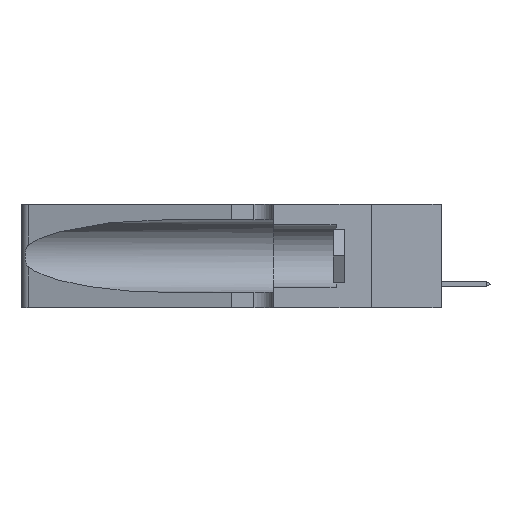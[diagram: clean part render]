
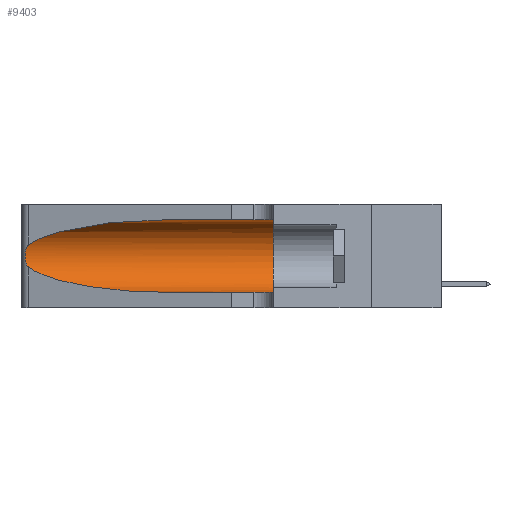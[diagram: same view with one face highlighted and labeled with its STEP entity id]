
A CAD part, left-side view. The second image highlights one B-rep face of the part: STEP entity #9403.
In plain terms, the highlighted cylindrical face has radius 3.308 mm (diameter 6.617 mm), a partial arc.
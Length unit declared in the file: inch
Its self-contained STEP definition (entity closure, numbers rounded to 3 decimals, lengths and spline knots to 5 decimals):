
#260 = DIRECTION ( 'NONE',  ( 0., 0., -1. ) ) ;
#383 = CARTESIAN_POINT ( 'NONE',  ( 0.1305, 0.35, 0.05475 ) ) ;
#609 = LINE ( 'NONE', #6390, #15550 ) ;
#777 = CARTESIAN_POINT ( 'NONE',  ( 0.2373, 1.15595, 0.28018 ) ) ;
#823 = EDGE_LOOP ( 'NONE', ( #16507, #5935, #15226, #9526, #3010, #2680 ) ) ;
#886 = EDGE_CURVE ( 'NONE', #3134, #11566, #5844, .T. ) ;
#1057 = AXIS2_PLACEMENT_3D ( 'NONE', #7533, #6177, #260 ) ;
#1418 = EDGE_CURVE ( 'NONE', #15803, #8553, #6634, .T. ) ;
#2193 = CARTESIAN_POINT ( 'NONE',  ( 0.25639, 1.23186, 0.15144 ) ) ;
#2226 = DIRECTION ( 'NONE',  ( 0., -1., 0. ) ) ;
#2521 = CYLINDRICAL_SURFACE ( 'NONE', #1057, 0.13025 ) ;
#2680 = ORIENTED_EDGE ( 'NONE', *, *, #7318, .F. ) ;
#3010 = ORIENTED_EDGE ( 'NONE', *, *, #6747, .F. ) ;
#3134 = VERTEX_POINT ( 'NONE', #3547 ) ;
#3521 = CARTESIAN_POINT ( 'NONE',  ( 0.25487, 1.22718, 0.22369 ) ) ;
#3547 = CARTESIAN_POINT ( 'NONE',  ( 0.25487, 1.22718, 0.14631 ) ) ;
#3558 = B_SPLINE_CURVE_WITH_KNOTS ( 'NONE', 3,
 ( #6538, #3743, #10888, #3803, #13723, #5171, #15155, #5228, #7777, #6603, #16568, #2193, #14972, #12322 ),
 .UNSPECIFIED., .F., .F.,
 ( 4, 2, 2, 2, 2, 2, 4 ),
 ( 0., 0.00027, 0.00053, 0.00107, 0.0016, 0.00187, 0.00214 ),
 .UNSPECIFIED. ) ;
#3738 = CARTESIAN_POINT ( 'NONE',  ( 0.1305, 0.72297, 0.05475 ) ) ;
#3743 = CARTESIAN_POINT ( 'NONE',  ( 0.25555, 1.22994, 0.2215 ) ) ;
#3803 = CARTESIAN_POINT ( 'NONE',  ( 0.25787, 1.23484, 0.2124 ) ) ;
#5097 = DIRECTION ( 'NONE',  ( 0., 0., 1. ) ) ;
#5171 = CARTESIAN_POINT ( 'NONE',  ( 0.26018, 1.23835, 0.19895 ) ) ;
#5228 = CARTESIAN_POINT ( 'NONE',  ( 0.26075, 1.23896, 0.178 ) ) ;
#5332 = CARTESIAN_POINT ( 'NONE',  ( 0.25487, 1.22718, 0.14631 ) ) ;
#5844 =( BOUNDED_CURVE ( )  B_SPLINE_CURVE ( 3, ( #5332, #10871, #15373, #6585 ),
 .UNSPECIFIED., .F., .F. ) 
 B_SPLINE_CURVE_WITH_KNOTS ( ( 4, 4 ),
 ( 3.44316, 4.71239 ),
 .UNSPECIFIED. ) 
 CURVE ( )  GEOMETRIC_REPRESENTATION_ITEM ( )  RATIONAL_B_SPLINE_CURVE ( ( 1., 0.87, 0.87, 1. ) ) 
 REPRESENTATION_ITEM ( '' )  );
#5935 = ORIENTED_EDGE ( 'NONE', *, *, #18329, .T. ) ;
#6177 = DIRECTION ( 'NONE',  ( 0., -1., 0. ) ) ;
#6390 = CARTESIAN_POINT ( 'NONE',  ( 0.1305, 1.61858, 0.31525 ) ) ;
#6538 = CARTESIAN_POINT ( 'NONE',  ( 0.25487, 1.22718, 0.22369 ) ) ;
#6585 = CARTESIAN_POINT ( 'NONE',  ( 0.1305, 0.72297, 0.05475 ) ) ;
#6603 = CARTESIAN_POINT ( 'NONE',  ( 0.25856, 1.23593, 0.16098 ) ) ;
#6634 =( BOUNDED_CURVE ( )  B_SPLINE_CURVE ( 3, ( #17713, #13750, #777, #3521 ),
 .UNSPECIFIED., .F., .F. ) 
 B_SPLINE_CURVE_WITH_KNOTS ( ( 4, 4 ),
 ( 1.5708, 2.84003 ),
 .UNSPECIFIED. ) 
 CURVE ( )  GEOMETRIC_REPRESENTATION_ITEM ( )  RATIONAL_B_SPLINE_CURVE ( ( 1., 0.87, 0.87, 1. ) ) 
 REPRESENTATION_ITEM ( '' )  );
#6747 = EDGE_CURVE ( 'NONE', #11287, #9374, #18190, .T. ) ;
#7244 = AXIS2_PLACEMENT_3D ( 'NONE', #16680, #8179, #5097 ) ;
#7318 = EDGE_CURVE ( 'NONE', #15803, #11287, #609, .T. ) ;
#7533 = CARTESIAN_POINT ( 'NONE',  ( 0.1305, 1.61858, 0.185 ) ) ;
#7777 = CARTESIAN_POINT ( 'NONE',  ( 0.26017, 1.23833, 0.17102 ) ) ;
#8179 = DIRECTION ( 'NONE',  ( 0., 1., 0. ) ) ;
#8553 = VERTEX_POINT ( 'NONE', #9485 ) ;
#8748 = CARTESIAN_POINT ( 'NONE',  ( 0.1305, 1.61858, 0.05475 ) ) ;
#8969 = FACE_OUTER_BOUND ( 'NONE', #823, .T. ) ;
#9374 = VERTEX_POINT ( 'NONE', #383 ) ;
#9403 = ADVANCED_FACE ( 'NONE', ( #8969 ), #2521, .F. ) ;
#9452 = VECTOR ( 'NONE', #15091, 39.37008 ) ;
#9485 = CARTESIAN_POINT ( 'NONE',  ( 0.25487, 1.22718, 0.22369 ) ) ;
#9526 = ORIENTED_EDGE ( 'NONE', *, *, #14032, .T. ) ;
#10871 = CARTESIAN_POINT ( 'NONE',  ( 0.2373, 1.15595, 0.08982 ) ) ;
#10888 = CARTESIAN_POINT ( 'NONE',  ( 0.25639, 1.23184, 0.21858 ) ) ;
#11287 = VERTEX_POINT ( 'NONE', #18428 ) ;
#11566 = VERTEX_POINT ( 'NONE', #3738 ) ;
#12322 = CARTESIAN_POINT ( 'NONE',  ( 0.25487, 1.22718, 0.14631 ) ) ;
#13723 = CARTESIAN_POINT ( 'NONE',  ( 0.25854, 1.2359, 0.20912 ) ) ;
#13750 = CARTESIAN_POINT ( 'NONE',  ( 0.18966, 0.96281, 0.31525 ) ) ;
#14032 = EDGE_CURVE ( 'NONE', #11566, #9374, #14180, .T. ) ;
#14180 = LINE ( 'NONE', #8748, #9452 ) ;
#14972 = CARTESIAN_POINT ( 'NONE',  ( 0.25555, 1.22993, 0.14849 ) ) ;
#15091 = DIRECTION ( 'NONE',  ( 0., -1., 0. ) ) ;
#15155 = CARTESIAN_POINT ( 'NONE',  ( 0.26075, 1.23896, 0.19203 ) ) ;
#15226 = ORIENTED_EDGE ( 'NONE', *, *, #886, .T. ) ;
#15373 = CARTESIAN_POINT ( 'NONE',  ( 0.18966, 0.96281, 0.05475 ) ) ;
#15550 = VECTOR ( 'NONE', #2226, 39.37008 ) ;
#15803 = VERTEX_POINT ( 'NONE', #17163 ) ;
#16507 = ORIENTED_EDGE ( 'NONE', *, *, #1418, .T. ) ;
#16568 = CARTESIAN_POINT ( 'NONE',  ( 0.25789, 1.23486, 0.15765 ) ) ;
#16680 = CARTESIAN_POINT ( 'NONE',  ( 0.1305, 0.35, 0.185 ) ) ;
#17163 = CARTESIAN_POINT ( 'NONE',  ( 0.1305, 0.72297, 0.31525 ) ) ;
#17713 = CARTESIAN_POINT ( 'NONE',  ( 0.1305, 0.72297, 0.31525 ) ) ;
#18190 = CIRCLE ( 'NONE', #7244, 0.13025 ) ;
#18329 = EDGE_CURVE ( 'NONE', #8553, #3134, #3558, .T. ) ;
#18428 = CARTESIAN_POINT ( 'NONE',  ( 0.1305, 0.35, 0.31525 ) ) ;
